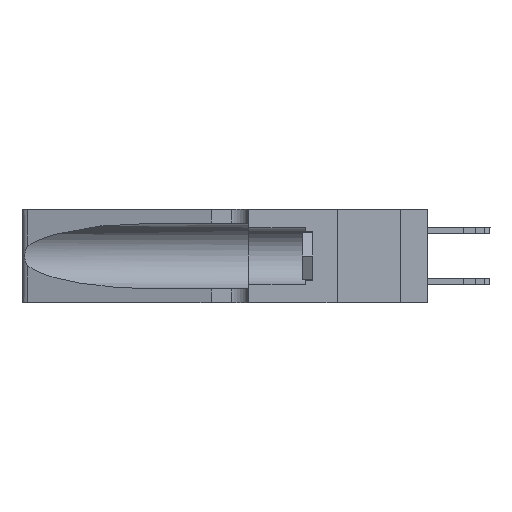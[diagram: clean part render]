
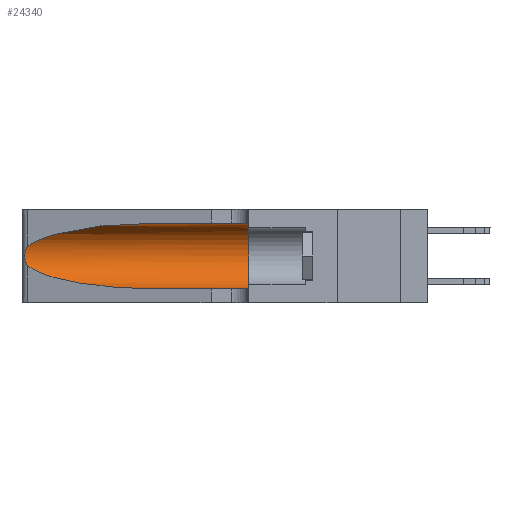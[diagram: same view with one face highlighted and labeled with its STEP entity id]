
A CAD part, left-side view. The second image highlights one B-rep face of the part: STEP entity #24340.
In plain terms, the highlighted cylindrical face has radius 3.308 mm (diameter 6.617 mm), a partial arc.
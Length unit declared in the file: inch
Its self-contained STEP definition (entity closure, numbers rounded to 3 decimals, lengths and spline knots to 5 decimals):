
#220 = CARTESIAN_POINT ( 'NONE',  ( 0.25487, 1.22718, 0.22369 ) ) ;
#494 = EDGE_CURVE ( 'NONE', #2145, #13306, #23113, .T. ) ;
#690 = AXIS2_PLACEMENT_3D ( 'NONE', #20044, #11678, #24408 ) ;
#899 = ORIENTED_EDGE ( 'NONE', *, *, #5273, .F. ) ;
#1306 = CIRCLE ( 'NONE', #24224, 0.13025 ) ;
#1437 = CARTESIAN_POINT ( 'NONE',  ( 0.26017, 1.23833, 0.17102 ) ) ;
#1752 = CARTESIAN_POINT ( 'NONE',  ( 0.2373, 1.15595, 0.08982 ) ) ;
#1778 = B_SPLINE_CURVE_WITH_KNOTS ( 'NONE', 3,
 ( #12881, #16850, #18967, #8609, #10573, #6384, #4352, #2353, #1437, #20458, #20131, #5807, #18664, #27116 ),
 .UNSPECIFIED., .F., .F.,
 ( 4, 2, 2, 2, 2, 2, 4 ),
 ( 0., 0.00027, 0.00053, 0.00107, 0.0016, 0.00187, 0.00214 ),
 .UNSPECIFIED. ) ;
#2145 = VERTEX_POINT ( 'NONE', #15599 ) ;
#2353 = CARTESIAN_POINT ( 'NONE',  ( 0.26075, 1.23896, 0.178 ) ) ;
#2473 = CARTESIAN_POINT ( 'NONE',  ( 0.2373, 1.15595, 0.28018 ) ) ;
#2990 = VECTOR ( 'NONE', #26960, 39.37008 ) ;
#3577 = EDGE_CURVE ( 'NONE', #16885, #10229, #16651, .T. ) ;
#4218 = EDGE_CURVE ( 'NONE', #13306, #16229, #1778, .T. ) ;
#4352 = CARTESIAN_POINT ( 'NONE',  ( 0.26075, 1.23896, 0.19203 ) ) ;
#5222 = CARTESIAN_POINT ( 'NONE',  ( 0.25487, 1.22718, 0.22369 ) ) ;
#5273 = EDGE_CURVE ( 'NONE', #2145, #23159, #23486, .T. ) ;
#5807 = CARTESIAN_POINT ( 'NONE',  ( 0.25639, 1.23186, 0.15144 ) ) ;
#5809 = EDGE_CURVE ( 'NONE', #23159, #10229, #1306, .T. ) ;
#6384 = CARTESIAN_POINT ( 'NONE',  ( 0.26018, 1.23835, 0.19895 ) ) ;
#7123 = CARTESIAN_POINT ( 'NONE',  ( 0.1305, 0.35, 0.185 ) ) ;
#7130 = ORIENTED_EDGE ( 'NONE', *, *, #14686, .T. ) ;
#8609 = CARTESIAN_POINT ( 'NONE',  ( 0.25787, 1.23484, 0.2124 ) ) ;
#9627 = EDGE_LOOP ( 'NONE', ( #21506, #22157, #7130, #12054, #13374, #899 ) ) ;
#9975 = CYLINDRICAL_SURFACE ( 'NONE', #690, 0.13025 ) ;
#10229 = VERTEX_POINT ( 'NONE', #12328 ) ;
#10515 = CARTESIAN_POINT ( 'NONE',  ( 0.1305, 0.72297, 0.05475 ) ) ;
#10573 = CARTESIAN_POINT ( 'NONE',  ( 0.25854, 1.2359, 0.20912 ) ) ;
#10879 = CARTESIAN_POINT ( 'NONE',  ( 0.1305, 0.72297, 0.31525 ) ) ;
#11016 = FACE_OUTER_BOUND ( 'NONE', #9627, .T. ) ;
#11351 = VECTOR ( 'NONE', #26001, 39.37008 ) ;
#11678 = DIRECTION ( 'NONE',  ( 0., -1., 0. ) ) ;
#11942 = DIRECTION ( 'NONE',  ( 0., 0., 1. ) ) ;
#12054 = ORIENTED_EDGE ( 'NONE', *, *, #3577, .T. ) ;
#12328 = CARTESIAN_POINT ( 'NONE',  ( 0.1305, 0.35, 0.05475 ) ) ;
#12514 = DIRECTION ( 'NONE',  ( 0., 1., 0. ) ) ;
#12881 = CARTESIAN_POINT ( 'NONE',  ( 0.25487, 1.22718, 0.22369 ) ) ;
#13306 = VERTEX_POINT ( 'NONE', #5222 ) ;
#13374 = ORIENTED_EDGE ( 'NONE', *, *, #5809, .F. ) ;
#13775 = CARTESIAN_POINT ( 'NONE',  ( 0.25487, 1.22718, 0.14631 ) ) ;
#14686 = EDGE_CURVE ( 'NONE', #16229, #16885, #27186, .T. ) ;
#15038 = CARTESIAN_POINT ( 'NONE',  ( 0.18966, 0.96281, 0.31525 ) ) ;
#15599 = CARTESIAN_POINT ( 'NONE',  ( 0.1305, 0.72297, 0.31525 ) ) ;
#16229 = VERTEX_POINT ( 'NONE', #13775 ) ;
#16651 = LINE ( 'NONE', #21734, #11351 ) ;
#16850 = CARTESIAN_POINT ( 'NONE',  ( 0.25555, 1.22994, 0.2215 ) ) ;
#16885 = VERTEX_POINT ( 'NONE', #16910 ) ;
#16910 = CARTESIAN_POINT ( 'NONE',  ( 0.1305, 0.72297, 0.05475 ) ) ;
#18664 = CARTESIAN_POINT ( 'NONE',  ( 0.25555, 1.22993, 0.14849 ) ) ;
#18967 = CARTESIAN_POINT ( 'NONE',  ( 0.25639, 1.23184, 0.21858 ) ) ;
#20044 = CARTESIAN_POINT ( 'NONE',  ( 0.1305, 1.61858, 0.185 ) ) ;
#20131 = CARTESIAN_POINT ( 'NONE',  ( 0.25789, 1.23486, 0.15765 ) ) ;
#20458 = CARTESIAN_POINT ( 'NONE',  ( 0.25856, 1.23593, 0.16098 ) ) ;
#20848 = CARTESIAN_POINT ( 'NONE',  ( 0.25487, 1.22718, 0.14631 ) ) ;
#21506 = ORIENTED_EDGE ( 'NONE', *, *, #494, .T. ) ;
#21734 = CARTESIAN_POINT ( 'NONE',  ( 0.1305, 1.61858, 0.05475 ) ) ;
#22157 = ORIENTED_EDGE ( 'NONE', *, *, #4218, .T. ) ;
#22264 = CARTESIAN_POINT ( 'NONE',  ( 0.1305, 1.61858, 0.31525 ) ) ;
#23113 =( BOUNDED_CURVE ( )  B_SPLINE_CURVE ( 3, ( #10879, #15038, #2473, #220 ),
 .UNSPECIFIED., .F., .T. ) 
 B_SPLINE_CURVE_WITH_KNOTS ( ( 4, 4 ),
 ( 1.5708, 2.84003 ),
 .UNSPECIFIED. ) 
 CURVE ( )  GEOMETRIC_REPRESENTATION_ITEM ( )  RATIONAL_B_SPLINE_CURVE ( ( 1., 0.87, 0.87, 1. ) ) 
 REPRESENTATION_ITEM ( '' )  );
#23159 = VERTEX_POINT ( 'NONE', #25827 ) ;
#23169 = CARTESIAN_POINT ( 'NONE',  ( 0.18966, 0.96281, 0.05475 ) ) ;
#23486 = LINE ( 'NONE', #22264, #2990 ) ;
#24224 = AXIS2_PLACEMENT_3D ( 'NONE', #7123, #12514, #11942 ) ;
#24340 = ADVANCED_FACE ( 'NONE', ( #11016 ), #9975, .F. ) ;
#24408 = DIRECTION ( 'NONE',  ( 0., 0., -1. ) ) ;
#25827 = CARTESIAN_POINT ( 'NONE',  ( 0.1305, 0.35, 0.31525 ) ) ;
#26001 = DIRECTION ( 'NONE',  ( 0., -1., 0. ) ) ;
#26960 = DIRECTION ( 'NONE',  ( 0., -1., 0. ) ) ;
#27116 = CARTESIAN_POINT ( 'NONE',  ( 0.25487, 1.22718, 0.14631 ) ) ;
#27186 =( BOUNDED_CURVE ( )  B_SPLINE_CURVE ( 3, ( #20848, #1752, #23169, #10515 ),
 .UNSPECIFIED., .F., .T. ) 
 B_SPLINE_CURVE_WITH_KNOTS ( ( 4, 4 ),
 ( 3.44316, 4.71239 ),
 .UNSPECIFIED. ) 
 CURVE ( )  GEOMETRIC_REPRESENTATION_ITEM ( )  RATIONAL_B_SPLINE_CURVE ( ( 1., 0.87, 0.87, 1. ) ) 
 REPRESENTATION_ITEM ( '' )  );
